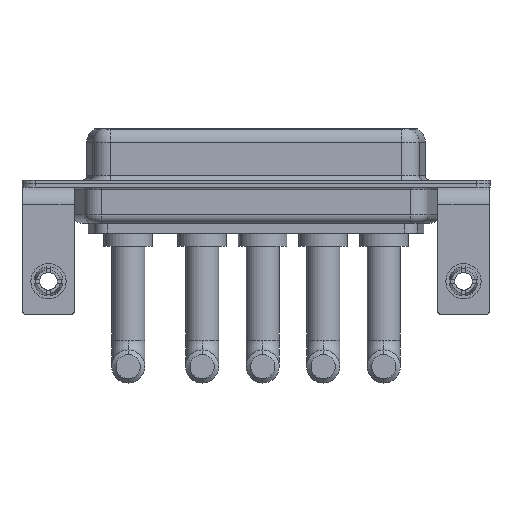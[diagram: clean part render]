
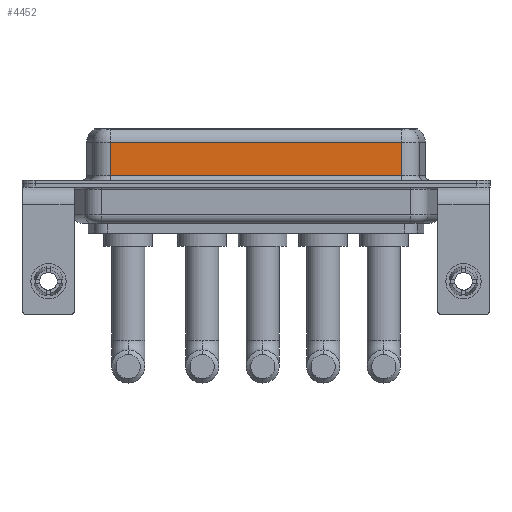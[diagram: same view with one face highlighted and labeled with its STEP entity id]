
A CAD part, front view. The second image highlights one B-rep face of the part: STEP entity #4452.
In plain terms, the highlighted planar face has unit normal (0, -1, 0).
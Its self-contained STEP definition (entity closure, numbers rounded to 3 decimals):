
#6 = VERTEX_POINT ( 'NONE', #9405 ) ;
#191 = LINE ( 'NONE', #10927, #12406 ) ;
#820 = EDGE_CURVE ( 'NONE', #6, #5977, #1985, .T. ) ;
#1474 = DIRECTION ( 'NONE',  ( 1., 0., 0. ) ) ;
#1774 = DIRECTION ( 'NONE',  ( 0., 0., -1. ) ) ;
#1955 = EDGE_CURVE ( 'NONE', #5977, #2924, #191, .T. ) ;
#1985 = LINE ( 'NONE', #11134, #9447 ) ;
#2209 = FACE_OUTER_BOUND ( 'NONE', #2500, .T. ) ;
#2500 = EDGE_LOOP ( 'NONE', ( #14840, #2561, #9857, #9530 ) ) ;
#2513 = EDGE_CURVE ( 'NONE', #7007, #2924, #14450, .T. ) ;
#2561 = ORIENTED_EDGE ( 'NONE', *, *, #9747, .T. ) ;
#2924 = VERTEX_POINT ( 'NONE', #3254 ) ;
#3254 = CARTESIAN_POINT ( 'NONE',  ( 40.037, -3.95, 0.9 ) ) ;
#3945 = AXIS2_PLACEMENT_3D ( 'NONE', #5650, #11573, #11500 ) ;
#4452 = ADVANCED_FACE ( 'NONE', ( #2209 ), #10213, .F. ) ;
#5289 = LINE ( 'NONE', #9930, #6562 ) ;
#5397 = CARTESIAN_POINT ( 'NONE',  ( 40.037, -3.95, 4.65 ) ) ;
#5650 = CARTESIAN_POINT ( 'NONE',  ( 40.037, -3.95, 6.4 ) ) ;
#5977 = VERTEX_POINT ( 'NONE', #13383 ) ;
#6562 = VECTOR ( 'NONE', #12147, 1000. ) ;
#7007 = VERTEX_POINT ( 'NONE', #5397 ) ;
#9405 = CARTESIAN_POINT ( 'NONE',  ( 7.013, -3.95, 4.65 ) ) ;
#9447 = VECTOR ( 'NONE', #10217, 1000. ) ;
#9530 = ORIENTED_EDGE ( 'NONE', *, *, #1955, .T. ) ;
#9747 = EDGE_CURVE ( 'NONE', #7007, #6, #5289, .T. ) ;
#9857 = ORIENTED_EDGE ( 'NONE', *, *, #820, .T. ) ;
#9930 = CARTESIAN_POINT ( 'NONE',  ( 40.037, -3.95, 4.65 ) ) ;
#10213 = PLANE ( 'NONE',  #3945 ) ;
#10217 = DIRECTION ( 'NONE',  ( 0., 0., -1. ) ) ;
#10927 = CARTESIAN_POINT ( 'NONE',  ( 40.037, -3.95, 0.9 ) ) ;
#11134 = CARTESIAN_POINT ( 'NONE',  ( 7.013, -3.95, 6.4 ) ) ;
#11500 = DIRECTION ( 'NONE',  ( 0., 0., 1. ) ) ;
#11573 = DIRECTION ( 'NONE',  ( 0., 1., 0. ) ) ;
#11964 = VECTOR ( 'NONE', #1774, 1000. ) ;
#12143 = CARTESIAN_POINT ( 'NONE',  ( 40.037, -3.95, 6.4 ) ) ;
#12147 = DIRECTION ( 'NONE',  ( -1., 0., 0. ) ) ;
#12406 = VECTOR ( 'NONE', #1474, 1000. ) ;
#13383 = CARTESIAN_POINT ( 'NONE',  ( 7.013, -3.95, 0.9 ) ) ;
#14450 = LINE ( 'NONE', #12143, #11964 ) ;
#14840 = ORIENTED_EDGE ( 'NONE', *, *, #2513, .F. ) ;
